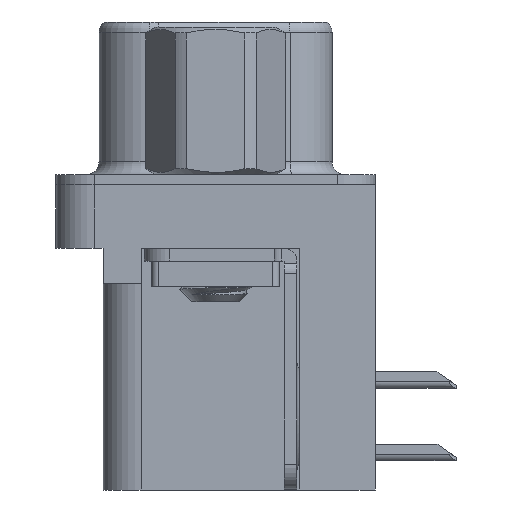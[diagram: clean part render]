
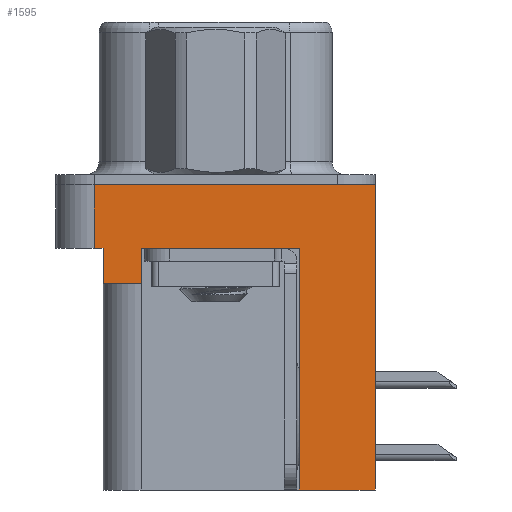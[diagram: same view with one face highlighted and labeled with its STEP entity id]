
A CAD part, left-side view. The second image highlights one B-rep face of the part: STEP entity #1595.
In plain terms, the highlighted planar face has unit normal (-1, 0, 0).
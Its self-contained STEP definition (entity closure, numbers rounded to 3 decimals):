
#11 = VERTEX_POINT ( 'NONE', #726 ) ;
#521 = VECTOR ( 'NONE', #24326, 1000. ) ;
#726 = CARTESIAN_POINT ( 'NONE',  ( -2.935, 4.425, -3.9 ) ) ;
#738 = DIRECTION ( 'NONE',  ( 0., 0., 1. ) ) ;
#760 = CARTESIAN_POINT ( 'NONE',  ( -2.935, 4.425, -3.9 ) ) ;
#963 = LINE ( 'NONE', #11362, #7881 ) ;
#1480 = ORIENTED_EDGE ( 'NONE', *, *, #10665, .T. ) ;
#1595 = ADVANCED_FACE ( 'NONE', ( #21827 ), #10303, .T. ) ;
#1674 = CARTESIAN_POINT ( 'NONE',  ( -2.935, 4.425, -2.5 ) ) ;
#1901 = DIRECTION ( 'NONE',  ( 0., 0., 1. ) ) ;
#2927 = CARTESIAN_POINT ( 'NONE',  ( -2.935, -6.275, -2.5 ) ) ;
#3065 = CARTESIAN_POINT ( 'NONE',  ( -2.935, 4.775, -2.5 ) ) ;
#3566 = ORIENTED_EDGE ( 'NONE', *, *, #13249, .F. ) ;
#3784 = ORIENTED_EDGE ( 'NONE', *, *, #10286, .T. ) ;
#4462 = LINE ( 'NONE', #5630, #10022 ) ;
#5093 = DIRECTION ( 'NONE',  ( 0., -1., 0. ) ) ;
#5130 = VERTEX_POINT ( 'NONE', #16855 ) ;
#5465 = EDGE_CURVE ( 'NONE', #18478, #14034, #21335, .T. ) ;
#5630 = CARTESIAN_POINT ( 'NONE',  ( -2.935, -6.275, -2.5 ) ) ;
#6003 = CARTESIAN_POINT ( 'NONE',  ( -2.935, -6.275, 0. ) ) ;
#6036 = VECTOR ( 'NONE', #19577, 1000. ) ;
#6245 = CARTESIAN_POINT ( 'NONE',  ( -2.935, 4.425, -3.9 ) ) ;
#6577 = CARTESIAN_POINT ( 'NONE',  ( -2.935, -6.275, 0. ) ) ;
#6760 = VERTEX_POINT ( 'NONE', #1674 ) ;
#7264 = EDGE_CURVE ( 'NONE', #11, #6760, #9650, .T. ) ;
#7881 = VECTOR ( 'NONE', #5093, 1000. ) ;
#7989 = LINE ( 'NONE', #16378, #21440 ) ;
#8275 = VECTOR ( 'NONE', #18518, 1000. ) ;
#8668 = EDGE_CURVE ( 'NONE', #5130, #11, #23622, .T. ) ;
#9138 = ORIENTED_EDGE ( 'NONE', *, *, #10874, .F. ) ;
#9547 = VERTEX_POINT ( 'NONE', #21969 ) ;
#9565 = EDGE_CURVE ( 'NONE', #16554, #9547, #18865, .T. ) ;
#9650 = LINE ( 'NONE', #6245, #521 ) ;
#9897 = VERTEX_POINT ( 'NONE', #6577 ) ;
#10022 = VECTOR ( 'NONE', #19408, 1000. ) ;
#10056 = DIRECTION ( 'NONE',  ( 0., -1., 0. ) ) ;
#10173 = ORIENTED_EDGE ( 'NONE', *, *, #7264, .F. ) ;
#10286 = EDGE_CURVE ( 'NONE', #16554, #9897, #17887, .T. ) ;
#10303 = PLANE ( 'NONE',  #18786 ) ;
#10665 = EDGE_CURVE ( 'NONE', #18478, #6760, #4462, .T. ) ;
#10752 = ORIENTED_EDGE ( 'NONE', *, *, #5465, .F. ) ;
#10804 = EDGE_LOOP ( 'NONE', ( #3566, #10752, #1480, #10173, #13843, #17990, #23175, #9138, #17805, #3784 ) ) ;
#10824 = CARTESIAN_POINT ( 'NONE',  ( -2.935, -6.275, -2.5 ) ) ;
#10874 = EDGE_CURVE ( 'NONE', #9547, #25870, #7989, .T. ) ;
#10916 = EDGE_CURVE ( 'NONE', #15700, #25870, #963, .T. ) ;
#11362 = CARTESIAN_POINT ( 'NONE',  ( -2.935, -6.275, -2.5 ) ) ;
#11692 = VECTOR ( 'NONE', #1901, 1000. ) ;
#12180 = CARTESIAN_POINT ( 'NONE',  ( -2.935, -3.295, -2.5 ) ) ;
#13165 = DIRECTION ( 'NONE',  ( 0., 0., 1. ) ) ;
#13249 = EDGE_CURVE ( 'NONE', #14034, #9897, #21196, .T. ) ;
#13829 = CARTESIAN_POINT ( 'NONE',  ( -2.935, 2.895, -2.5 ) ) ;
#13843 = ORIENTED_EDGE ( 'NONE', *, *, #8668, .F. ) ;
#13844 = CARTESIAN_POINT ( 'NONE',  ( -2.935, 2.895, -3.9 ) ) ;
#14034 = VERTEX_POINT ( 'NONE', #14150 ) ;
#14150 = CARTESIAN_POINT ( 'NONE',  ( -2.935, 4.775, 0. ) ) ;
#14491 = VECTOR ( 'NONE', #22121, 1000. ) ;
#14513 = LINE ( 'NONE', #13844, #11692 ) ;
#15700 = VERTEX_POINT ( 'NONE', #13829 ) ;
#16378 = CARTESIAN_POINT ( 'NONE',  ( -2.935, -3.295, -12. ) ) ;
#16554 = VERTEX_POINT ( 'NONE', #20682 ) ;
#16855 = CARTESIAN_POINT ( 'NONE',  ( -2.935, 2.895, -3.9 ) ) ;
#16866 = DIRECTION ( 'NONE',  ( -1., 0., 0. ) ) ;
#17805 = ORIENTED_EDGE ( 'NONE', *, *, #9565, .F. ) ;
#17887 = LINE ( 'NONE', #10824, #20698 ) ;
#17990 = ORIENTED_EDGE ( 'NONE', *, *, #19622, .T. ) ;
#18478 = VERTEX_POINT ( 'NONE', #3065 ) ;
#18518 = DIRECTION ( 'NONE',  ( 0., 1., 0. ) ) ;
#18786 = AXIS2_PLACEMENT_3D ( 'NONE', #2927, #16866, #20969 ) ;
#18865 = LINE ( 'NONE', #19981, #14491 ) ;
#19408 = DIRECTION ( 'NONE',  ( 0., -1., 0. ) ) ;
#19577 = DIRECTION ( 'NONE',  ( 0., 0., 1. ) ) ;
#19622 = EDGE_CURVE ( 'NONE', #5130, #15700, #14513, .T. ) ;
#19981 = CARTESIAN_POINT ( 'NONE',  ( -2.935, -3.295, -12. ) ) ;
#20260 = VECTOR ( 'NONE', #10056, 1000. ) ;
#20682 = CARTESIAN_POINT ( 'NONE',  ( -2.935, -6.275, -12. ) ) ;
#20698 = VECTOR ( 'NONE', #738, 1000. ) ;
#20969 = DIRECTION ( 'NONE',  ( 0., 0., 1. ) ) ;
#21196 = LINE ( 'NONE', #6003, #20260 ) ;
#21335 = LINE ( 'NONE', #21409, #6036 ) ;
#21409 = CARTESIAN_POINT ( 'NONE',  ( -2.935, 4.775, -2.5 ) ) ;
#21440 = VECTOR ( 'NONE', #13165, 1000. ) ;
#21827 = FACE_OUTER_BOUND ( 'NONE', #10804, .T. ) ;
#21969 = CARTESIAN_POINT ( 'NONE',  ( -2.935, -3.295, -12. ) ) ;
#22121 = DIRECTION ( 'NONE',  ( 0., 1., 0. ) ) ;
#23175 = ORIENTED_EDGE ( 'NONE', *, *, #10916, .T. ) ;
#23622 = LINE ( 'NONE', #760, #8275 ) ;
#24326 = DIRECTION ( 'NONE',  ( 0., 0., 1. ) ) ;
#25870 = VERTEX_POINT ( 'NONE', #12180 ) ;
